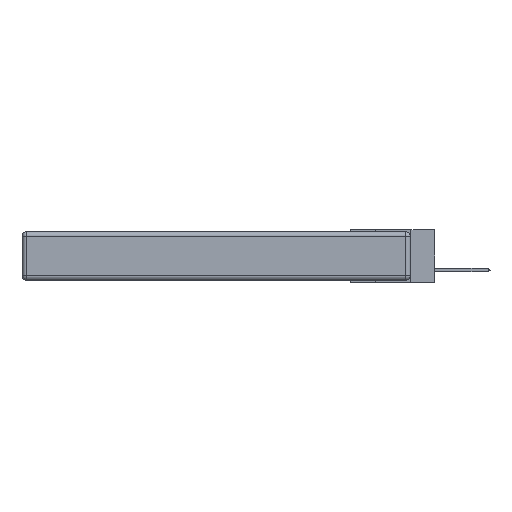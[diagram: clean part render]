
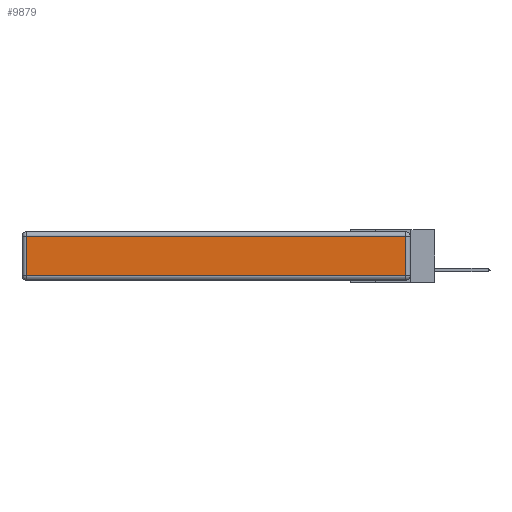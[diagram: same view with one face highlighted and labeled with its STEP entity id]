
A CAD part, left-side view. The second image highlights one B-rep face of the part: STEP entity #9879.
In plain terms, the highlighted planar face has unit normal (-1, 0, 0).
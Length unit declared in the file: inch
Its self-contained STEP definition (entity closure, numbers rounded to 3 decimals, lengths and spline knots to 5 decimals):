
#106 = LINE ( 'NONE', #15189, #2177 ) ;
#372 = LINE ( 'NONE', #10949, #16757 ) ;
#1550 = CARTESIAN_POINT ( 'NONE',  ( 0., 0.03, -0.343 ) ) ;
#2054 = LINE ( 'NONE', #2740, #4705 ) ;
#2177 = VECTOR ( 'NONE', #4558, 39.37008 ) ;
#2422 = PLANE ( 'NONE',  #8152 ) ;
#2740 = CARTESIAN_POINT ( 'NONE',  ( 0., 0., -0.313 ) ) ;
#2855 = ORIENTED_EDGE ( 'NONE', *, *, #9290, .T. ) ;
#3167 = VERTEX_POINT ( 'NONE', #15793 ) ;
#3330 = VECTOR ( 'NONE', #13361, 39.37008 ) ;
#3377 = ORIENTED_EDGE ( 'NONE', *, *, #9634, .T. ) ;
#3645 = EDGE_CURVE ( 'NONE', #3167, #14165, #14123, .T. ) ;
#3676 = DIRECTION ( 'NONE',  ( -1., 0., 0. ) ) ;
#4541 = VERTEX_POINT ( 'NONE', #7654 ) ;
#4552 = CARTESIAN_POINT ( 'NONE',  ( 0., 0.03, -0.03 ) ) ;
#4558 = DIRECTION ( 'NONE',  ( 0., 1., 0. ) ) ;
#4705 = VECTOR ( 'NONE', #7857, 39.37008 ) ;
#5082 = ORIENTED_EDGE ( 'NONE', *, *, #11420, .T. ) ;
#6913 = FACE_OUTER_BOUND ( 'NONE', #14212, .T. ) ;
#7654 = CARTESIAN_POINT ( 'NONE',  ( 0., 2.72, -0.313 ) ) ;
#7857 = DIRECTION ( 'NONE',  ( 0., -1., 0. ) ) ;
#8152 = AXIS2_PLACEMENT_3D ( 'NONE', #15507, #3676, #10317 ) ;
#9290 = EDGE_CURVE ( 'NONE', #4541, #3167, #2054, .T. ) ;
#9634 = EDGE_CURVE ( 'NONE', #10518, #4541, #372, .T. ) ;
#9879 = ADVANCED_FACE ( 'NONE', ( #6913 ), #2422, .T. ) ;
#10317 = DIRECTION ( 'NONE',  ( 0., 0., 1. ) ) ;
#10483 = ORIENTED_EDGE ( 'NONE', *, *, #3645, .T. ) ;
#10518 = VERTEX_POINT ( 'NONE', #14442 ) ;
#10949 = CARTESIAN_POINT ( 'NONE',  ( 0., 2.72, -0.343 ) ) ;
#11420 = EDGE_CURVE ( 'NONE', #14165, #10518, #106, .T. ) ;
#12253 = DIRECTION ( 'NONE',  ( 0., 0., -1. ) ) ;
#13361 = DIRECTION ( 'NONE',  ( 0., 0., 1. ) ) ;
#14123 = LINE ( 'NONE', #1550, #3330 ) ;
#14165 = VERTEX_POINT ( 'NONE', #4552 ) ;
#14212 = EDGE_LOOP ( 'NONE', ( #2855, #10483, #5082, #3377 ) ) ;
#14442 = CARTESIAN_POINT ( 'NONE',  ( 0., 2.72, -0.03 ) ) ;
#15189 = CARTESIAN_POINT ( 'NONE',  ( 0., 2.75, -0.03 ) ) ;
#15507 = CARTESIAN_POINT ( 'NONE',  ( 0., 0., -0.343 ) ) ;
#15793 = CARTESIAN_POINT ( 'NONE',  ( 0., 0.03, -0.313 ) ) ;
#16757 = VECTOR ( 'NONE', #12253, 39.37008 ) ;
